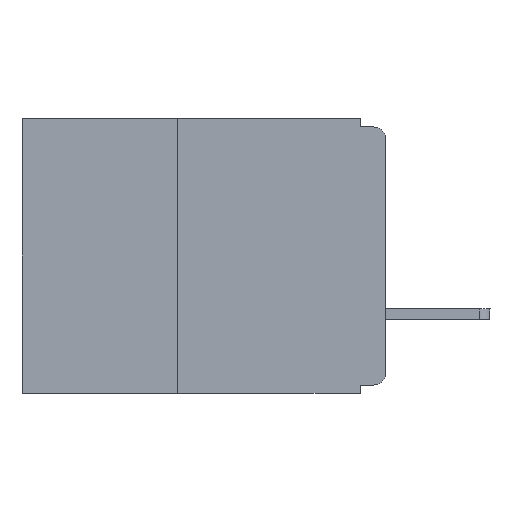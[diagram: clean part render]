
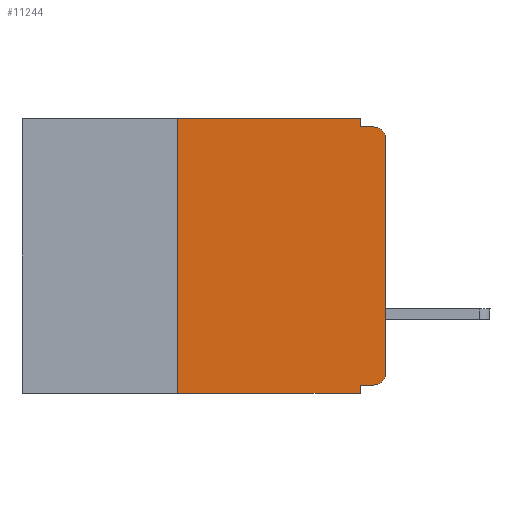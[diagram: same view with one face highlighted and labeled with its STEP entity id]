
A CAD part, left-side view. The second image highlights one B-rep face of the part: STEP entity #11244.
In plain terms, the highlighted planar face has unit normal (-1, 0, 0).
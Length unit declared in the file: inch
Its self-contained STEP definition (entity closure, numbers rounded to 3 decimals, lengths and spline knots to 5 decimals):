
#31 = EDGE_CURVE ( 'NONE', #210, #8516, #1375, .T. ) ;
#210 = VERTEX_POINT ( 'NONE', #10090 ) ;
#414 = ORIENTED_EDGE ( 'NONE', *, *, #5839, .F. ) ;
#467 = CARTESIAN_POINT ( 'NONE',  ( 0., 0., -0.305 ) ) ;
#680 = AXIS2_PLACEMENT_3D ( 'NONE', #13937, #3642, #6406 ) ;
#682 = EDGE_CURVE ( 'NONE', #14969, #10251, #10689, .T. ) ;
#1375 = CIRCLE ( 'NONE', #680, 0.015 ) ;
#1496 = LINE ( 'NONE', #9132, #14590 ) ;
#1736 = DIRECTION ( 'NONE',  ( 0., 0., 1. ) ) ;
#1743 = CARTESIAN_POINT ( 'NONE',  ( 0., 0., -0.025 ) ) ;
#2035 = EDGE_CURVE ( 'NONE', #5276, #7328, #9042, .T. ) ;
#2229 = DIRECTION ( 'NONE',  ( 0., 0., -1. ) ) ;
#2729 = DIRECTION ( 'NONE',  ( 0., -1., 0. ) ) ;
#3565 = DIRECTION ( 'NONE',  ( 0., 1., 0. ) ) ;
#3642 = DIRECTION ( 'NONE',  ( -1., 0., 0. ) ) ;
#4155 = DIRECTION ( 'NONE',  ( 0., 0., -1. ) ) ;
#4612 = CIRCLE ( 'NONE', #12507, 0.015 ) ;
#4900 = VECTOR ( 'NONE', #3565, 39.37008 ) ;
#5046 = LINE ( 'NONE', #13011, #9002 ) ;
#5168 = VERTEX_POINT ( 'NONE', #1743 ) ;
#5276 = VERTEX_POINT ( 'NONE', #16227 ) ;
#5839 = EDGE_CURVE ( 'NONE', #210, #13607, #9072, .T. ) ;
#5966 = VECTOR ( 'NONE', #14119, 39.37008 ) ;
#5993 = ORIENTED_EDGE ( 'NONE', *, *, #682, .T. ) ;
#6067 = CARTESIAN_POINT ( 'NONE',  ( 0., 0.25, -0.33 ) ) ;
#6364 = ORIENTED_EDGE ( 'NONE', *, *, #8428, .T. ) ;
#6406 = DIRECTION ( 'NONE',  ( 0., 0., -1. ) ) ;
#7263 = EDGE_CURVE ( 'NONE', #14969, #10758, #1496, .T. ) ;
#7328 = VERTEX_POINT ( 'NONE', #10074 ) ;
#7405 = ORIENTED_EDGE ( 'NONE', *, *, #31, .T. ) ;
#7664 = CARTESIAN_POINT ( 'NONE',  ( 0., 0.25, 0. ) ) ;
#7705 = CARTESIAN_POINT ( 'NONE',  ( 0., 0.437, 0. ) ) ;
#7826 = CARTESIAN_POINT ( 'NONE',  ( 0., 0.437, -0.33 ) ) ;
#7905 = ORIENTED_EDGE ( 'NONE', *, *, #12187, .F. ) ;
#8056 = ORIENTED_EDGE ( 'NONE', *, *, #2035, .F. ) ;
#8142 = DIRECTION ( 'NONE',  ( 0., 0., -1. ) ) ;
#8428 = EDGE_CURVE ( 'NONE', #8516, #5168, #5046, .T. ) ;
#8449 = ORIENTED_EDGE ( 'NONE', *, *, #16048, .F. ) ;
#8516 = VERTEX_POINT ( 'NONE', #467 ) ;
#8568 = AXIS2_PLACEMENT_3D ( 'NONE', #11832, #9321, #8142 ) ;
#8886 = CARTESIAN_POINT ( 'NONE',  ( 0., 0., -0.01 ) ) ;
#9002 = VECTOR ( 'NONE', #1736, 39.37008 ) ;
#9042 = LINE ( 'NONE', #8886, #14999 ) ;
#9072 = LINE ( 'NONE', #9925, #4900 ) ;
#9132 = CARTESIAN_POINT ( 'NONE',  ( 0., 0.25, -0.33 ) ) ;
#9151 = DIRECTION ( 'NONE',  ( 0., -1., 0. ) ) ;
#9321 = DIRECTION ( 'NONE',  ( 1., 0., 0. ) ) ;
#9333 = LINE ( 'NONE', #7705, #5966 ) ;
#9341 = ORIENTED_EDGE ( 'NONE', *, *, #7263, .F. ) ;
#9417 = EDGE_CURVE ( 'NONE', #5168, #7328, #4612, .T. ) ;
#9734 = CARTESIAN_POINT ( 'NONE',  ( 0., 0.031, -0.33 ) ) ;
#9826 = CARTESIAN_POINT ( 'NONE',  ( 0., 0.031, 0. ) ) ;
#9925 = CARTESIAN_POINT ( 'NONE',  ( 0., 0., -0.32 ) ) ;
#9949 = CARTESIAN_POINT ( 'NONE',  ( 0., 0.031, -0.33 ) ) ;
#10074 = CARTESIAN_POINT ( 'NONE',  ( 0., 0.015, -0.01 ) ) ;
#10090 = CARTESIAN_POINT ( 'NONE',  ( 0., 0.015, -0.32 ) ) ;
#10251 = VERTEX_POINT ( 'NONE', #9949 ) ;
#10426 = DIRECTION ( 'NONE',  ( -1., 0., 0. ) ) ;
#10689 = LINE ( 'NONE', #7826, #13267 ) ;
#10758 = VERTEX_POINT ( 'NONE', #7664 ) ;
#11023 = DIRECTION ( 'NONE',  ( 0., 0., -1. ) ) ;
#11061 = LINE ( 'NONE', #9734, #12257 ) ;
#11244 = ADVANCED_FACE ( 'NONE', ( #11280 ), #15710, .F. ) ;
#11280 = FACE_OUTER_BOUND ( 'NONE', #14832, .T. ) ;
#11760 = DIRECTION ( 'NONE',  ( 0., 0., 1. ) ) ;
#11832 = CARTESIAN_POINT ( 'NONE',  ( 0., 0.437, 0. ) ) ;
#11838 = ORIENTED_EDGE ( 'NONE', *, *, #11946, .F. ) ;
#11946 = EDGE_CURVE ( 'NONE', #13607, #10251, #11061, .T. ) ;
#11979 = CARTESIAN_POINT ( 'NONE',  ( 0., 0.031, -0.32 ) ) ;
#12187 = EDGE_CURVE ( 'NONE', #14943, #5276, #14196, .T. ) ;
#12257 = VECTOR ( 'NONE', #11023, 39.37008 ) ;
#12507 = AXIS2_PLACEMENT_3D ( 'NONE', #15378, #10426, #4155 ) ;
#13011 = CARTESIAN_POINT ( 'NONE',  ( 0., 0., 0. ) ) ;
#13267 = VECTOR ( 'NONE', #9151, 39.37008 ) ;
#13607 = VERTEX_POINT ( 'NONE', #11979 ) ;
#13937 = CARTESIAN_POINT ( 'NONE',  ( 0., 0.015, -0.305 ) ) ;
#14119 = DIRECTION ( 'NONE',  ( 0., -1., 0. ) ) ;
#14196 = LINE ( 'NONE', #15108, #15618 ) ;
#14590 = VECTOR ( 'NONE', #11760, 39.37008 ) ;
#14832 = EDGE_LOOP ( 'NONE', ( #6364, #16109, #8056, #7905, #8449, #9341, #5993, #11838, #414, #7405 ) ) ;
#14943 = VERTEX_POINT ( 'NONE', #9826 ) ;
#14969 = VERTEX_POINT ( 'NONE', #6067 ) ;
#14999 = VECTOR ( 'NONE', #2729, 39.37008 ) ;
#15108 = CARTESIAN_POINT ( 'NONE',  ( 0., 0.031, 0. ) ) ;
#15378 = CARTESIAN_POINT ( 'NONE',  ( 0., 0.015, -0.025 ) ) ;
#15618 = VECTOR ( 'NONE', #2229, 39.37008 ) ;
#15710 = PLANE ( 'NONE',  #8568 ) ;
#16048 = EDGE_CURVE ( 'NONE', #10758, #14943, #9333, .T. ) ;
#16109 = ORIENTED_EDGE ( 'NONE', *, *, #9417, .T. ) ;
#16227 = CARTESIAN_POINT ( 'NONE',  ( 0., 0.031, -0.01 ) ) ;
